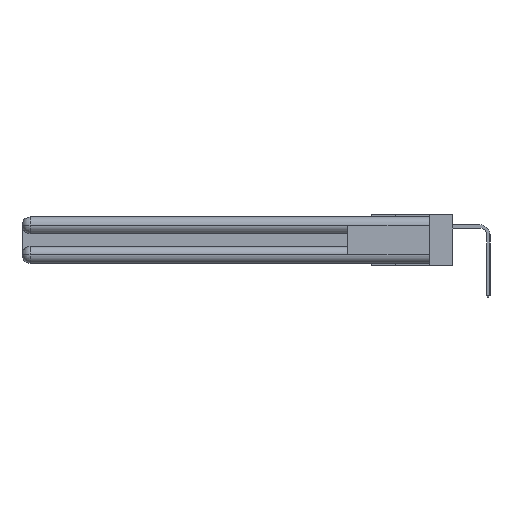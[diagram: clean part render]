
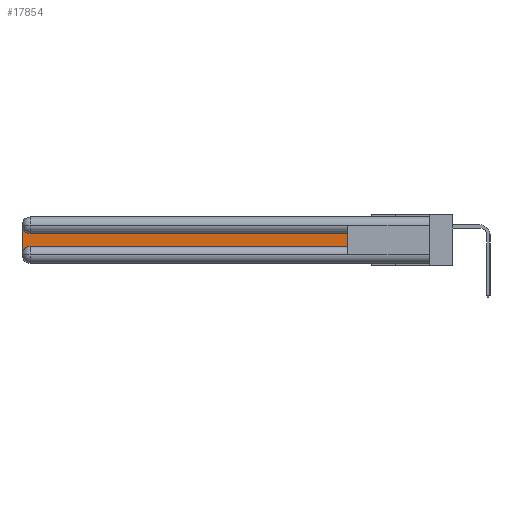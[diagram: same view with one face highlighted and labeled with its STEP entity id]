
A CAD part, left-side view. The second image highlights one B-rep face of the part: STEP entity #17854.
In plain terms, the highlighted planar face has unit normal (-1, 0, 0).
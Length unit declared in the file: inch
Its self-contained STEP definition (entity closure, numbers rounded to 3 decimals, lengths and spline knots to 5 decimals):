
#470 = DIRECTION ( 'NONE',  ( 0., 0., -1. ) ) ;
#1304 = EDGE_CURVE ( 'NONE', #21397, #20681, #28403, .T. ) ;
#3684 = VERTEX_POINT ( 'NONE', #4103 ) ;
#3704 = CARTESIAN_POINT ( 'NONE',  ( 0.075, 2.94, -0.2175 ) ) ;
#3998 = VECTOR ( 'NONE', #23198, 39.37008 ) ;
#4103 = CARTESIAN_POINT ( 'NONE',  ( 0.075, 0.6, -0.1225 ) ) ;
#4625 = ORIENTED_EDGE ( 'NONE', *, *, #8897, .T. ) ;
#4827 = ORIENTED_EDGE ( 'NONE', *, *, #24689, .T. ) ;
#4850 = CIRCLE ( 'NONE', #28133, 0.06 ) ;
#5891 = DIRECTION ( 'NONE',  ( 0., 0., -1. ) ) ;
#6420 = EDGE_CURVE ( 'NONE', #7132, #24465, #4850, .T. ) ;
#6906 = EDGE_LOOP ( 'NONE', ( #4827, #9946, #4625, #26712, #28607, #27509 ) ) ;
#7132 = VERTEX_POINT ( 'NONE', #22850 ) ;
#7140 = CARTESIAN_POINT ( 'NONE',  ( 0.075, 3., -0.2175 ) ) ;
#7233 = DIRECTION ( 'NONE',  ( 0., 0., -1. ) ) ;
#8451 = LINE ( 'NONE', #14670, #3998 ) ;
#8569 = CARTESIAN_POINT ( 'NONE',  ( 0.075, 3., -0.0625 ) ) ;
#8897 = EDGE_CURVE ( 'NONE', #24465, #21397, #25382, .T. ) ;
#8967 = EDGE_CURVE ( 'NONE', #30226, #3684, #8451, .T. ) ;
#9946 = ORIENTED_EDGE ( 'NONE', *, *, #6420, .T. ) ;
#10609 = PLANE ( 'NONE',  #20493 ) ;
#10792 = CARTESIAN_POINT ( 'NONE',  ( 0.075, 3., -0.2775 ) ) ;
#11348 = VECTOR ( 'NONE', #25959, 39.37008 ) ;
#12367 = CARTESIAN_POINT ( 'NONE',  ( 0.075, 2.94, -0.0625 ) ) ;
#13012 = FACE_OUTER_BOUND ( 'NONE', #6906, .T. ) ;
#14670 = CARTESIAN_POINT ( 'NONE',  ( 0.075, 0.6, -0.2175 ) ) ;
#14821 = DIRECTION ( 'NONE',  ( 1., 0., 0. ) ) ;
#15574 = DIRECTION ( 'NONE',  ( 1., 0., 0. ) ) ;
#16010 = VECTOR ( 'NONE', #28230, 39.37008 ) ;
#17274 = CARTESIAN_POINT ( 'NONE',  ( 0.075, 0.6, -0.2175 ) ) ;
#17633 = DIRECTION ( 'NONE',  ( 1., 0., 0. ) ) ;
#17854 = ADVANCED_FACE ( 'NONE', ( #13012 ), #10609, .F. ) ;
#19007 = VECTOR ( 'NONE', #7233, 39.37008 ) ;
#19630 = LINE ( 'NONE', #21192, #11348 ) ;
#19779 = LINE ( 'NONE', #30805, #16010 ) ;
#20493 = AXIS2_PLACEMENT_3D ( 'NONE', #25312, #15574, #5891 ) ;
#20681 = VERTEX_POINT ( 'NONE', #3704 ) ;
#21192 = CARTESIAN_POINT ( 'NONE',  ( 0.075, 0.6, -0.2175 ) ) ;
#21254 = AXIS2_PLACEMENT_3D ( 'NONE', #22483, #17633, #24652 ) ;
#21397 = VERTEX_POINT ( 'NONE', #10792 ) ;
#22483 = CARTESIAN_POINT ( 'NONE',  ( 0.075, 2.94, -0.2775 ) ) ;
#22850 = CARTESIAN_POINT ( 'NONE',  ( 0.075, 2.94, -0.1225 ) ) ;
#23198 = DIRECTION ( 'NONE',  ( 0., 0., 1. ) ) ;
#24465 = VERTEX_POINT ( 'NONE', #8569 ) ;
#24652 = DIRECTION ( 'NONE',  ( 0., 0., -1. ) ) ;
#24689 = EDGE_CURVE ( 'NONE', #3684, #7132, #19779, .T. ) ;
#25312 = CARTESIAN_POINT ( 'NONE',  ( 0.075, 3., -0.1225 ) ) ;
#25382 = LINE ( 'NONE', #7140, #19007 ) ;
#25959 = DIRECTION ( 'NONE',  ( 0., -1., 0. ) ) ;
#26712 = ORIENTED_EDGE ( 'NONE', *, *, #1304, .T. ) ;
#27509 = ORIENTED_EDGE ( 'NONE', *, *, #8967, .T. ) ;
#28133 = AXIS2_PLACEMENT_3D ( 'NONE', #12367, #14821, #470 ) ;
#28230 = DIRECTION ( 'NONE',  ( 0., 1., 0. ) ) ;
#28403 = CIRCLE ( 'NONE', #21254, 0.06 ) ;
#28607 = ORIENTED_EDGE ( 'NONE', *, *, #30718, .T. ) ;
#30226 = VERTEX_POINT ( 'NONE', #17274 ) ;
#30718 = EDGE_CURVE ( 'NONE', #20681, #30226, #19630, .T. ) ;
#30805 = CARTESIAN_POINT ( 'NONE',  ( 0.075, 0.6, -0.1225 ) ) ;
